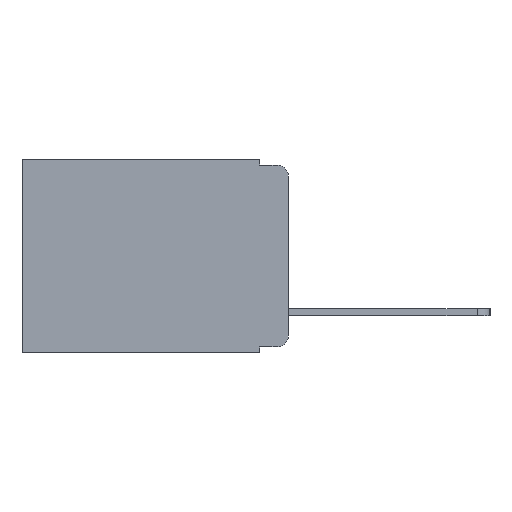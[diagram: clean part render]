
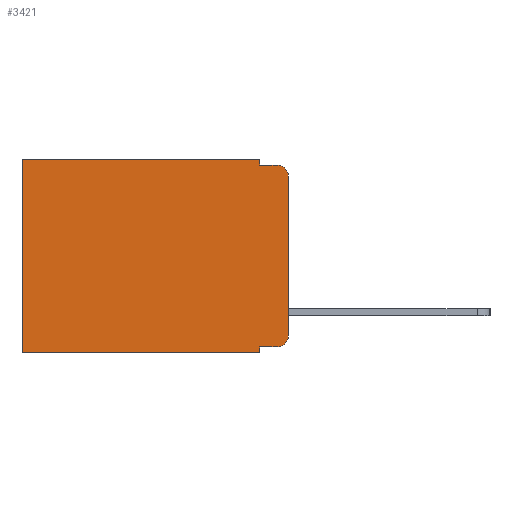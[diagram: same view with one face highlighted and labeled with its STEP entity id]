
A CAD part, left-side view. The second image highlights one B-rep face of the part: STEP entity #3421.
In plain terms, the highlighted planar face has unit normal (-1, 0, 0).
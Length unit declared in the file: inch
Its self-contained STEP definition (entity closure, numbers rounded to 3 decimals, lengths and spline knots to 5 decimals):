
#96 = EDGE_LOOP ( 'NONE', ( #6894, #7251, #2815, #681, #2945, #3532, #3377, #8045, #10518, #3845 ) ) ;
#447 = CARTESIAN_POINT ( 'NONE',  ( 0.298, 0.051, -0.333 ) ) ;
#536 = VECTOR ( 'NONE', #9910, 39.37008 ) ;
#681 = ORIENTED_EDGE ( 'NONE', *, *, #6464, .F. ) ;
#723 = VERTEX_POINT ( 'NONE', #6957 ) ;
#817 = DIRECTION ( 'NONE',  ( -1., 0., 0. ) ) ;
#1372 = CARTESIAN_POINT ( 'NONE',  ( 0.298, 0.051, -0.01 ) ) ;
#1637 = CARTESIAN_POINT ( 'NONE',  ( 0.298, 0., -0.03 ) ) ;
#1792 = FACE_OUTER_BOUND ( 'NONE', #96, .T. ) ;
#1988 = VERTEX_POINT ( 'NONE', #8955 ) ;
#2000 = VECTOR ( 'NONE', #8379, 39.37008 ) ;
#2005 = DIRECTION ( 'NONE',  ( 0., 0., -1. ) ) ;
#2289 = VERTEX_POINT ( 'NONE', #10381 ) ;
#2321 = DIRECTION ( 'NONE',  ( 0., 0., -1. ) ) ;
#2710 = LINE ( 'NONE', #5905, #9175 ) ;
#2815 = ORIENTED_EDGE ( 'NONE', *, *, #4633, .F. ) ;
#2872 = CIRCLE ( 'NONE', #7904, 0.02 ) ;
#2945 = ORIENTED_EDGE ( 'NONE', *, *, #9512, .T. ) ;
#3068 = VERTEX_POINT ( 'NONE', #7583 ) ;
#3167 = DIRECTION ( 'NONE',  ( 0., 0., -1. ) ) ;
#3175 = DIRECTION ( 'NONE',  ( 1., 0., 0. ) ) ;
#3190 = PLANE ( 'NONE',  #4488 ) ;
#3266 = CARTESIAN_POINT ( 'NONE',  ( 0.298, 0.473, 0. ) ) ;
#3377 = ORIENTED_EDGE ( 'NONE', *, *, #9132, .F. ) ;
#3416 = CARTESIAN_POINT ( 'NONE',  ( 0.298, 0.051, 0. ) ) ;
#3421 = ADVANCED_FACE ( 'NONE', ( #1792 ), #3190, .F. ) ;
#3532 = ORIENTED_EDGE ( 'NONE', *, *, #6917, .T. ) ;
#3845 = ORIENTED_EDGE ( 'NONE', *, *, #5715, .T. ) ;
#4226 = EDGE_CURVE ( 'NONE', #5771, #2289, #2710, .T. ) ;
#4243 = LINE ( 'NONE', #3416, #10263 ) ;
#4488 = AXIS2_PLACEMENT_3D ( 'NONE', #7847, #3175, #3167 ) ;
#4594 = VECTOR ( 'NONE', #7455, 39.37008 ) ;
#4598 = EDGE_CURVE ( 'NONE', #5771, #723, #2872, .T. ) ;
#4633 = EDGE_CURVE ( 'NONE', #10479, #723, #10917, .T. ) ;
#4811 = DIRECTION ( 'NONE',  ( 0., 1., 0. ) ) ;
#4842 = CARTESIAN_POINT ( 'NONE',  ( 0.298, 0.02, -0.03 ) ) ;
#5140 = VERTEX_POINT ( 'NONE', #6343 ) ;
#5144 = CARTESIAN_POINT ( 'NONE',  ( 0.298, 0.051, 0. ) ) ;
#5700 = DIRECTION ( 'NONE',  ( 0., 0., -1. ) ) ;
#5715 = EDGE_CURVE ( 'NONE', #3068, #2289, #6088, .T. ) ;
#5736 = VERTEX_POINT ( 'NONE', #11001 ) ;
#5771 = VERTEX_POINT ( 'NONE', #1637 ) ;
#5857 = VERTEX_POINT ( 'NONE', #7841 ) ;
#5905 = CARTESIAN_POINT ( 'NONE',  ( 0.298, 0., 0. ) ) ;
#6031 = VECTOR ( 'NONE', #4811, 39.37008 ) ;
#6077 = LINE ( 'NONE', #8060, #10143 ) ;
#6088 = CIRCLE ( 'NONE', #8221, 0.02 ) ;
#6242 = CARTESIAN_POINT ( 'NONE',  ( 0.298, 0.02, -0.313 ) ) ;
#6343 = CARTESIAN_POINT ( 'NONE',  ( 0.298, 0.473, -0.343 ) ) ;
#6464 = EDGE_CURVE ( 'NONE', #8623, #10479, #6077, .T. ) ;
#6851 = LINE ( 'NONE', #7428, #4594 ) ;
#6894 = ORIENTED_EDGE ( 'NONE', *, *, #4226, .F. ) ;
#6917 = EDGE_CURVE ( 'NONE', #1988, #5140, #9109, .T. ) ;
#6957 = CARTESIAN_POINT ( 'NONE',  ( 0.298, 0.02, -0.01 ) ) ;
#6989 = EDGE_CURVE ( 'NONE', #5857, #5736, #4243, .T. ) ;
#7078 = DIRECTION ( 'NONE',  ( 0., 0., -1. ) ) ;
#7127 = EDGE_CURVE ( 'NONE', #5857, #3068, #9761, .T. ) ;
#7157 = CARTESIAN_POINT ( 'NONE',  ( 0.298, 0.051, -0.01 ) ) ;
#7251 = ORIENTED_EDGE ( 'NONE', *, *, #4598, .T. ) ;
#7299 = DIRECTION ( 'NONE',  ( -1., 0., 0. ) ) ;
#7428 = CARTESIAN_POINT ( 'NONE',  ( 0.298, 0., -0.343 ) ) ;
#7455 = DIRECTION ( 'NONE',  ( 0., 1., 0. ) ) ;
#7583 = CARTESIAN_POINT ( 'NONE',  ( 0.298, 0.02, -0.333 ) ) ;
#7841 = CARTESIAN_POINT ( 'NONE',  ( 0.298, 0.051, -0.333 ) ) ;
#7847 = CARTESIAN_POINT ( 'NONE',  ( 0.298, 0., 0. ) ) ;
#7904 = AXIS2_PLACEMENT_3D ( 'NONE', #4842, #7299, #2005 ) ;
#8045 = ORIENTED_EDGE ( 'NONE', *, *, #6989, .F. ) ;
#8060 = CARTESIAN_POINT ( 'NONE',  ( 0.298, 0.051, 0. ) ) ;
#8124 = CARTESIAN_POINT ( 'NONE',  ( 0.298, 0., 0. ) ) ;
#8218 = LINE ( 'NONE', #8124, #6031 ) ;
#8221 = AXIS2_PLACEMENT_3D ( 'NONE', #6242, #817, #7078 ) ;
#8224 = DIRECTION ( 'NONE',  ( 0., 0., -1. ) ) ;
#8379 = DIRECTION ( 'NONE',  ( 0., 0., -1. ) ) ;
#8623 = VERTEX_POINT ( 'NONE', #5144 ) ;
#8803 = VECTOR ( 'NONE', #10937, 39.37008 ) ;
#8955 = CARTESIAN_POINT ( 'NONE',  ( 0.298, 0.473, 0. ) ) ;
#9109 = LINE ( 'NONE', #3266, #2000 ) ;
#9132 = EDGE_CURVE ( 'NONE', #5736, #5140, #6851, .T. ) ;
#9175 = VECTOR ( 'NONE', #8224, 39.37008 ) ;
#9512 = EDGE_CURVE ( 'NONE', #8623, #1988, #8218, .T. ) ;
#9761 = LINE ( 'NONE', #447, #536 ) ;
#9910 = DIRECTION ( 'NONE',  ( 0., -1., 0. ) ) ;
#10143 = VECTOR ( 'NONE', #5700, 39.37008 ) ;
#10263 = VECTOR ( 'NONE', #2321, 39.37008 ) ;
#10381 = CARTESIAN_POINT ( 'NONE',  ( 0.298, 0., -0.313 ) ) ;
#10479 = VERTEX_POINT ( 'NONE', #1372 ) ;
#10518 = ORIENTED_EDGE ( 'NONE', *, *, #7127, .T. ) ;
#10917 = LINE ( 'NONE', #7157, #8803 ) ;
#10937 = DIRECTION ( 'NONE',  ( 0., -1., 0. ) ) ;
#11001 = CARTESIAN_POINT ( 'NONE',  ( 0.298, 0.051, -0.343 ) ) ;
